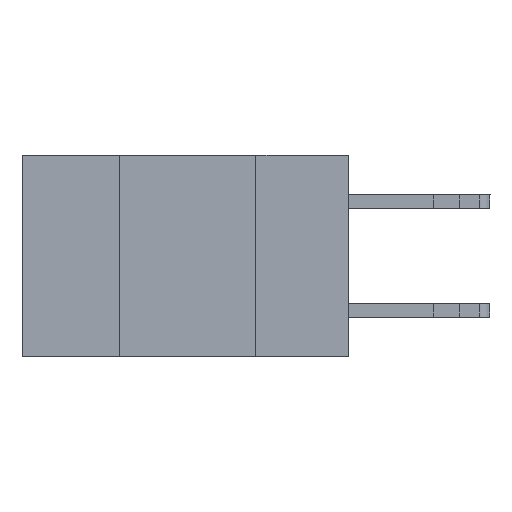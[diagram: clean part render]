
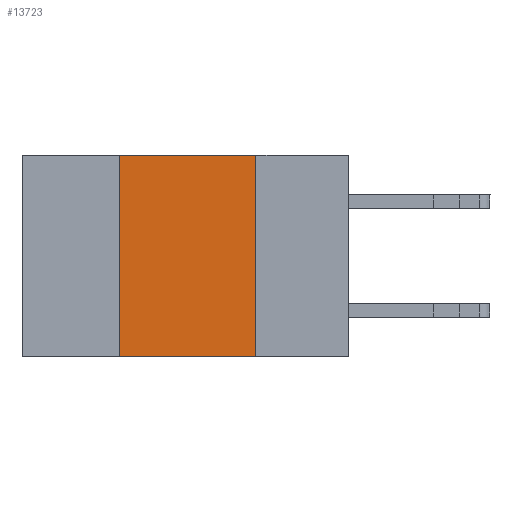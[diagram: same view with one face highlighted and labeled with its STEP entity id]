
A CAD part, left-side view. The second image highlights one B-rep face of the part: STEP entity #13723.
In plain terms, the highlighted planar face has unit normal (-1, 0, 0).
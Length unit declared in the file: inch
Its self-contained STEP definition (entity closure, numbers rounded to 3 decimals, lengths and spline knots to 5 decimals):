
#431 = CARTESIAN_POINT ( 'NONE',  ( 0., 0.17, -0.37 ) ) ;
#505 = CARTESIAN_POINT ( 'NONE',  ( 0., 0.6, 0. ) ) ;
#648 = LINE ( 'NONE', #3612, #9308 ) ;
#1582 = VECTOR ( 'NONE', #1829, 39.37008 ) ;
#1829 = DIRECTION ( 'NONE',  ( 0., 0., -1. ) ) ;
#3301 = ORIENTED_EDGE ( 'NONE', *, *, #11932, .T. ) ;
#3612 = CARTESIAN_POINT ( 'NONE',  ( 0., 0.6, -0.37 ) ) ;
#5321 = VERTEX_POINT ( 'NONE', #12223 ) ;
#5569 = LINE ( 'NONE', #505, #6106 ) ;
#5665 = CARTESIAN_POINT ( 'NONE',  ( 0., 0.17, 0. ) ) ;
#5872 = ORIENTED_EDGE ( 'NONE', *, *, #8822, .F. ) ;
#5914 = LINE ( 'NONE', #5665, #1582 ) ;
#6106 = VECTOR ( 'NONE', #12042, 39.37008 ) ;
#6373 = DIRECTION ( 'NONE',  ( 1., 0., 0. ) ) ;
#6512 = ORIENTED_EDGE ( 'NONE', *, *, #11544, .F. ) ;
#7205 = VERTEX_POINT ( 'NONE', #12222 ) ;
#8441 = VECTOR ( 'NONE', #9189, 39.37008 ) ;
#8488 = VERTEX_POINT ( 'NONE', #14848 ) ;
#8511 = ORIENTED_EDGE ( 'NONE', *, *, #16670, .F. ) ;
#8689 = EDGE_LOOP ( 'NONE', ( #8511, #5872, #6512, #3301 ) ) ;
#8822 = EDGE_CURVE ( 'NONE', #8488, #7205, #5569, .T. ) ;
#9189 = DIRECTION ( 'NONE',  ( 0., 0., 1. ) ) ;
#9308 = VECTOR ( 'NONE', #14120, 39.37008 ) ;
#10514 = FACE_OUTER_BOUND ( 'NONE', #8689, .T. ) ;
#10553 = LINE ( 'NONE', #12951, #8441 ) ;
#11544 = EDGE_CURVE ( 'NONE', #5321, #8488, #10553, .T. ) ;
#11732 = DIRECTION ( 'NONE',  ( 0., 0., -1. ) ) ;
#11932 = EDGE_CURVE ( 'NONE', #5321, #16652, #648, .T. ) ;
#12042 = DIRECTION ( 'NONE',  ( 0., -1., 0. ) ) ;
#12222 = CARTESIAN_POINT ( 'NONE',  ( 0., 0.17, 0. ) ) ;
#12223 = CARTESIAN_POINT ( 'NONE',  ( 0., 0.42, -0.37 ) ) ;
#12914 = CARTESIAN_POINT ( 'NONE',  ( 0., 0.6, 0. ) ) ;
#12951 = CARTESIAN_POINT ( 'NONE',  ( 0., 0.42, 0. ) ) ;
#13457 = AXIS2_PLACEMENT_3D ( 'NONE', #12914, #6373, #11732 ) ;
#13723 = ADVANCED_FACE ( 'NONE', ( #10514 ), #14356, .F. ) ;
#14120 = DIRECTION ( 'NONE',  ( 0., -1., 0. ) ) ;
#14356 = PLANE ( 'NONE',  #13457 ) ;
#14848 = CARTESIAN_POINT ( 'NONE',  ( 0., 0.42, 0. ) ) ;
#16652 = VERTEX_POINT ( 'NONE', #431 ) ;
#16670 = EDGE_CURVE ( 'NONE', #7205, #16652, #5914, .T. ) ;
